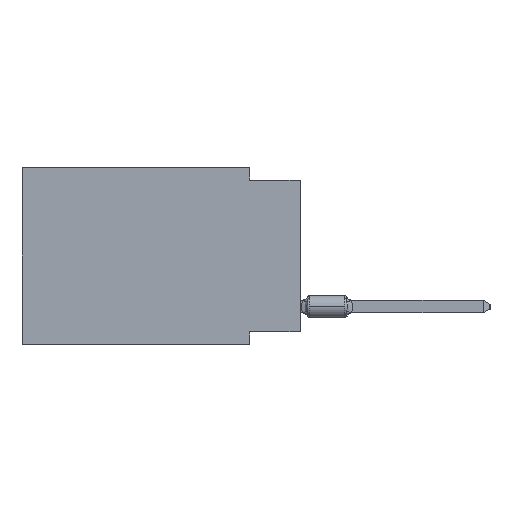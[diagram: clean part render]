
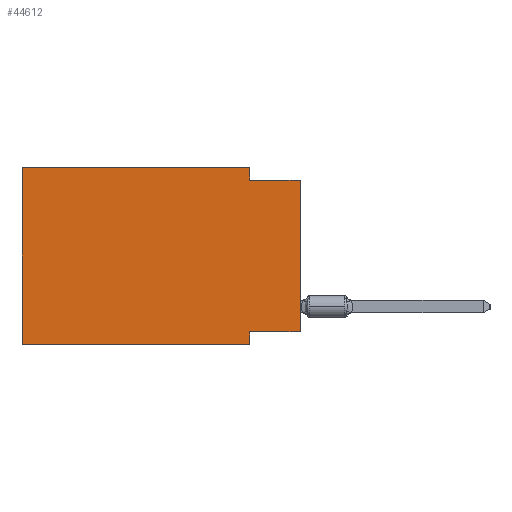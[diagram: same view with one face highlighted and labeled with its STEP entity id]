
A CAD part, left-side view. The second image highlights one B-rep face of the part: STEP entity #44612.
In plain terms, the highlighted planar face has unit normal (-1, 0, 0).
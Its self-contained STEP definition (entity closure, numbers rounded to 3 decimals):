
#777 = VERTEX_POINT ( 'NONE', #95566 ) ;
#3127 = LINE ( 'NONE', #58842, #24313 ) ;
#3571 = ORIENTED_EDGE ( 'NONE', *, *, #6392, .T. ) ;
#4103 = DIRECTION ( 'NONE',  ( 0., -1., 0. ) ) ;
#4165 = VERTEX_POINT ( 'NONE', #34305 ) ;
#6392 = EDGE_CURVE ( 'NONE', #15054, #777, #95098, .T. ) ;
#7324 = CARTESIAN_POINT ( 'NONE',  ( 0., 2.54, -0.635 ) ) ;
#8681 = VECTOR ( 'NONE', #27763, 1000. ) ;
#11186 = VECTOR ( 'NONE', #39915, 1000. ) ;
#12919 = LINE ( 'NONE', #36450, #8681 ) ;
#13496 = CARTESIAN_POINT ( 'NONE',  ( 0., 13.97, 0. ) ) ;
#14765 = VERTEX_POINT ( 'NONE', #7324 ) ;
#15054 = VERTEX_POINT ( 'NONE', #43509 ) ;
#15617 = EDGE_LOOP ( 'NONE', ( #3571, #28805, #95446, #34161, #64184, #33791, #81935, #17303 ) ) ;
#17303 = ORIENTED_EDGE ( 'NONE', *, *, #66223, .F. ) ;
#20452 = DIRECTION ( 'NONE',  ( 0., -1., 0. ) ) ;
#22204 = DIRECTION ( 'NONE',  ( 0., 0., 1. ) ) ;
#24313 = VECTOR ( 'NONE', #57846, 1000. ) ;
#25124 = CARTESIAN_POINT ( 'NONE',  ( 0., 13.97, 0. ) ) ;
#26638 = LINE ( 'NONE', #57831, #30998 ) ;
#27763 = DIRECTION ( 'NONE',  ( 0., 0., -1. ) ) ;
#28805 = ORIENTED_EDGE ( 'NONE', *, *, #30476, .F. ) ;
#30476 = EDGE_CURVE ( 'NONE', #14765, #777, #59320, .T. ) ;
#30998 = VECTOR ( 'NONE', #88995, 1000. ) ;
#33166 = VERTEX_POINT ( 'NONE', #74841 ) ;
#33791 = ORIENTED_EDGE ( 'NONE', *, *, #90144, .T. ) ;
#34161 = ORIENTED_EDGE ( 'NONE', *, *, #34608, .F. ) ;
#34305 = CARTESIAN_POINT ( 'NONE',  ( 0., 2.54, -8.89 ) ) ;
#34608 = EDGE_CURVE ( 'NONE', #44204, #94889, #3127, .T. ) ;
#36450 = CARTESIAN_POINT ( 'NONE',  ( 0., 2.54, -8.89 ) ) ;
#37830 = PLANE ( 'NONE',  #65519 ) ;
#39915 = DIRECTION ( 'NONE',  ( 0., 0., 1. ) ) ;
#42169 = LINE ( 'NONE', #88690, #97182 ) ;
#43454 = DIRECTION ( 'NONE',  ( 0., 0., -1. ) ) ;
#43509 = CARTESIAN_POINT ( 'NONE',  ( 0., 0., -8.255 ) ) ;
#44204 = VERTEX_POINT ( 'NONE', #25124 ) ;
#44612 = ADVANCED_FACE ( 'NONE', ( #99179 ), #37830, .F. ) ;
#45490 = DIRECTION ( 'NONE',  ( 1., 0., 0. ) ) ;
#48130 = VECTOR ( 'NONE', #22204, 1000. ) ;
#50079 = CARTESIAN_POINT ( 'NONE',  ( 0., 13.97, -8.89 ) ) ;
#55288 = VECTOR ( 'NONE', #20452, 1000. ) ;
#57831 = CARTESIAN_POINT ( 'NONE',  ( 0., 2.54, 0. ) ) ;
#57846 = DIRECTION ( 'NONE',  ( 0., -1., 0. ) ) ;
#58805 = CARTESIAN_POINT ( 'NONE',  ( 0., 13.97, -8.89 ) ) ;
#58842 = CARTESIAN_POINT ( 'NONE',  ( 0., 13.97, 0. ) ) ;
#59320 = LINE ( 'NONE', #65503, #59845 ) ;
#59845 = VECTOR ( 'NONE', #4103, 1000. ) ;
#60326 = CARTESIAN_POINT ( 'NONE',  ( 0., 13.97, 0. ) ) ;
#62076 = LINE ( 'NONE', #13496, #48130 ) ;
#64184 = ORIENTED_EDGE ( 'NONE', *, *, #84785, .F. ) ;
#65503 = CARTESIAN_POINT ( 'NONE',  ( 0., 0., -0.635 ) ) ;
#65519 = AXIS2_PLACEMENT_3D ( 'NONE', #60326, #45490, #43454 ) ;
#66223 = EDGE_CURVE ( 'NONE', #15054, #33166, #42169, .T. ) ;
#70749 = VERTEX_POINT ( 'NONE', #50079 ) ;
#72661 = LINE ( 'NONE', #58805, #55288 ) ;
#74841 = CARTESIAN_POINT ( 'NONE',  ( 0., 2.54, -8.255 ) ) ;
#78269 = CARTESIAN_POINT ( 'NONE',  ( 0., 0., 0. ) ) ;
#81935 = ORIENTED_EDGE ( 'NONE', *, *, #98872, .F. ) ;
#82019 = DIRECTION ( 'NONE',  ( 0., 1., 0. ) ) ;
#84785 = EDGE_CURVE ( 'NONE', #70749, #44204, #62076, .T. ) ;
#88690 = CARTESIAN_POINT ( 'NONE',  ( 0., 0., -8.255 ) ) ;
#88995 = DIRECTION ( 'NONE',  ( 0., 0., -1. ) ) ;
#89622 = CARTESIAN_POINT ( 'NONE',  ( 0., 2.54, 0. ) ) ;
#90144 = EDGE_CURVE ( 'NONE', #70749, #4165, #72661, .T. ) ;
#92981 = EDGE_CURVE ( 'NONE', #94889, #14765, #26638, .T. ) ;
#94889 = VERTEX_POINT ( 'NONE', #89622 ) ;
#95098 = LINE ( 'NONE', #78269, #11186 ) ;
#95446 = ORIENTED_EDGE ( 'NONE', *, *, #92981, .F. ) ;
#95566 = CARTESIAN_POINT ( 'NONE',  ( 0., 0., -0.635 ) ) ;
#97182 = VECTOR ( 'NONE', #82019, 1000. ) ;
#98872 = EDGE_CURVE ( 'NONE', #33166, #4165, #12919, .T. ) ;
#99179 = FACE_OUTER_BOUND ( 'NONE', #15617, .T. ) ;
